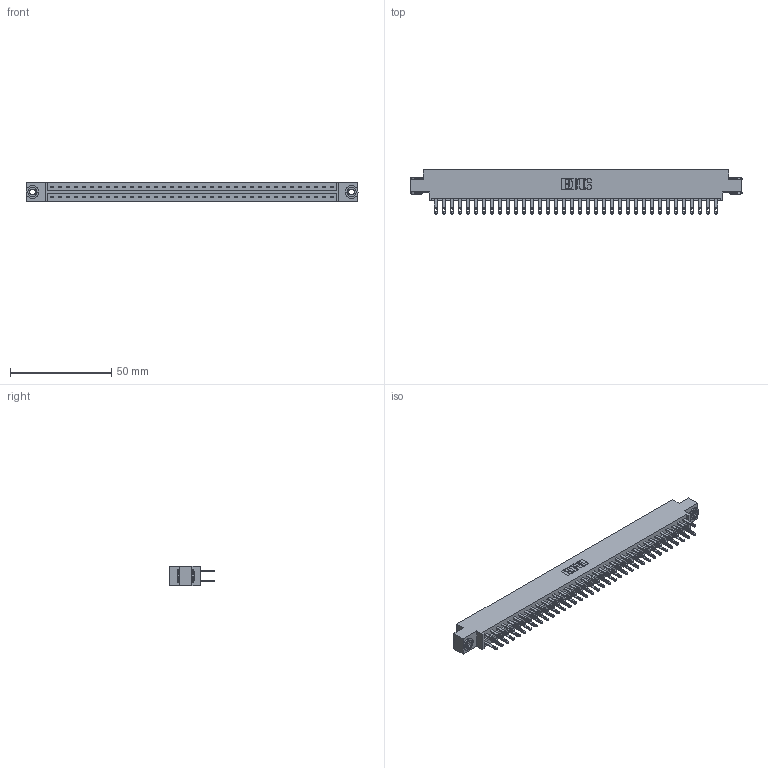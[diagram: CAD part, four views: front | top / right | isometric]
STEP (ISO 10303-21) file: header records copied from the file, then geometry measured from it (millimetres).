
FILE_DESCRIPTION (( 'STEP AP203' ), '1' );
FILE_NAME ('833-072-500-803.STEP', '2020-06-05T13:34:21', ( '' ), ( '' ), 'SwSTEP 2.0', 'SolidWorks 2020', '' );
FILE_SCHEMA (( 'CONFIG_CONTROL_DESIGN' ));
Length unit declared in the file: inch
Products named in the file (4): 345-292-001_345-293-100; 345-250-002_345-250-002-102; 833 Part_Offset - .156 Dia - TH; 833-072-500-803
Assembly tree (75 placements, depth 2):
  833-072-500-803
    833 Part_Offset - .156 Dia - TH
    345-292-001_345-293-100  x72
    345-250-002_345-250-002-102  x2
Bounding box: 164.19 x 21.85 x 9.4 mm (x, y, z)
Volume: 16717.9 mm3; surface area: 20934.3 mm2
Topology: 75 solids, 75 shells, 3612 faces, 10983 edges, 7318 vertices
Faces by surface type: plane 2244, cylinder 1360, cone 8
Entity records: 24648 total; most frequent: CARTESIAN_POINT 4069, ORIENTED_EDGE 3998, DIRECTION 3521, EDGE_CURVE 1999, LINE 1843, VECTOR 1843, VERTEX_POINT 1330, AXIS2_PLACEMENT_3D 839
